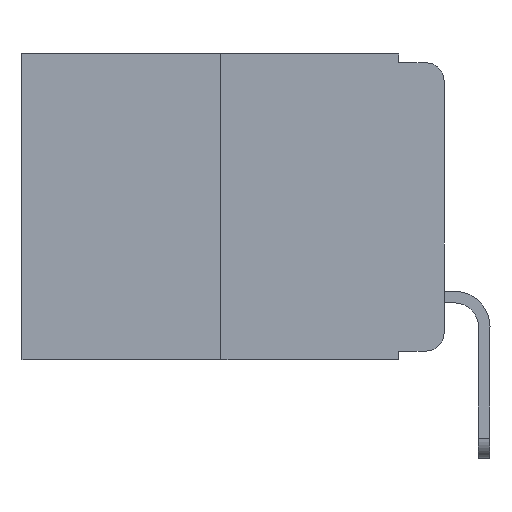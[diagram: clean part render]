
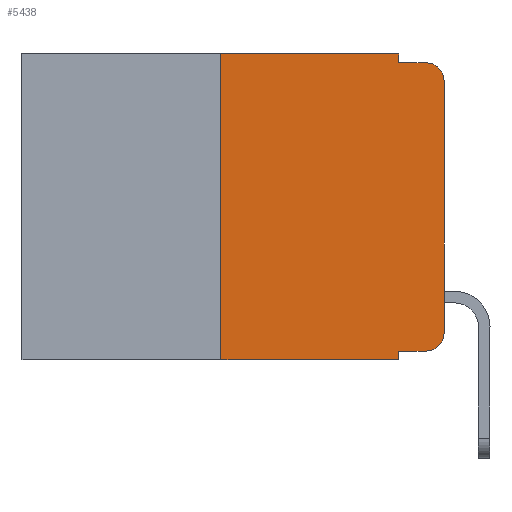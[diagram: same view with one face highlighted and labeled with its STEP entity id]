
A CAD part, left-side view. The second image highlights one B-rep face of the part: STEP entity #5438.
In plain terms, the highlighted planar face has unit normal (-1, 0, 0).
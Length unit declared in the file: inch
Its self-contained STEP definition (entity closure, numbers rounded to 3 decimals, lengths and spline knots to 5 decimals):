
#16 = DIRECTION ( 'NONE',  ( 0., 0., -1. ) ) ;
#187 = CARTESIAN_POINT ( 'NONE',  ( 0., 0., -0.313 ) ) ;
#477 = ORIENTED_EDGE ( 'NONE', *, *, #481, .T. ) ;
#481 = EDGE_CURVE ( 'NONE', #2038, #12820, #4282, .T. ) ;
#696 = EDGE_CURVE ( 'NONE', #2451, #9400, #4997, .T. ) ;
#844 = VERTEX_POINT ( 'NONE', #4598 ) ;
#1097 = CARTESIAN_POINT ( 'NONE',  ( 0., 0.473, -0.343 ) ) ;
#1273 = ORIENTED_EDGE ( 'NONE', *, *, #2085, .T. ) ;
#1280 = VECTOR ( 'NONE', #8300, 39.37008 ) ;
#1400 = LINE ( 'NONE', #3022, #12144 ) ;
#1419 = CARTESIAN_POINT ( 'NONE',  ( 0., 0.473, 0. ) ) ;
#1587 = CARTESIAN_POINT ( 'NONE',  ( 0., 0.25, -0.343 ) ) ;
#1633 = VECTOR ( 'NONE', #10096, 39.37008 ) ;
#1708 = CARTESIAN_POINT ( 'NONE',  ( 0., 0.051, 0. ) ) ;
#1951 = ORIENTED_EDGE ( 'NONE', *, *, #5269, .F. ) ;
#2038 = VERTEX_POINT ( 'NONE', #187 ) ;
#2085 = EDGE_CURVE ( 'NONE', #12820, #3923, #8723, .T. ) ;
#2230 = VERTEX_POINT ( 'NONE', #1587 ) ;
#2451 = VERTEX_POINT ( 'NONE', #7808 ) ;
#2529 = LINE ( 'NONE', #4290, #1633 ) ;
#2653 = VECTOR ( 'NONE', #7726, 39.37008 ) ;
#3007 = FACE_OUTER_BOUND ( 'NONE', #12797, .T. ) ;
#3022 = CARTESIAN_POINT ( 'NONE',  ( 0., 0.051, -0.333 ) ) ;
#3183 = AXIS2_PLACEMENT_3D ( 'NONE', #14115, #6069, #3643 ) ;
#3369 = LINE ( 'NONE', #1419, #11816 ) ;
#3457 = ORIENTED_EDGE ( 'NONE', *, *, #11152, .T. ) ;
#3540 = CARTESIAN_POINT ( 'NONE',  ( 0., 0.02, -0.313 ) ) ;
#3643 = DIRECTION ( 'NONE',  ( 0., 0., -1. ) ) ;
#3923 = VERTEX_POINT ( 'NONE', #4450 ) ;
#4162 = ORIENTED_EDGE ( 'NONE', *, *, #10431, .F. ) ;
#4205 = ORIENTED_EDGE ( 'NONE', *, *, #12530, .F. ) ;
#4282 = LINE ( 'NONE', #14617, #2653 ) ;
#4290 = CARTESIAN_POINT ( 'NONE',  ( 0., 0.051, -0.01 ) ) ;
#4398 = EDGE_CURVE ( 'NONE', #7217, #3923, #2529, .T. ) ;
#4450 = CARTESIAN_POINT ( 'NONE',  ( 0., 0.02, -0.01 ) ) ;
#4598 = CARTESIAN_POINT ( 'NONE',  ( 0., 0.02, -0.333 ) ) ;
#4603 = PLANE ( 'NONE',  #7050 ) ;
#4630 = CIRCLE ( 'NONE', #14713, 0.02 ) ;
#4679 = CARTESIAN_POINT ( 'NONE',  ( 0., 0.25, 0. ) ) ;
#4997 = LINE ( 'NONE', #1708, #12148 ) ;
#5269 = EDGE_CURVE ( 'NONE', #13619, #13014, #3369, .T. ) ;
#5276 = CARTESIAN_POINT ( 'NONE',  ( 0., 0.25, 0. ) ) ;
#5438 = ADVANCED_FACE ( 'NONE', ( #3007 ), #4603, .F. ) ;
#5814 = EDGE_CURVE ( 'NONE', #844, #2038, #4630, .T. ) ;
#6069 = DIRECTION ( 'NONE',  ( -1., 0., 0. ) ) ;
#6144 = LINE ( 'NONE', #4679, #1280 ) ;
#6895 = DIRECTION ( 'NONE',  ( 1., 0., 0. ) ) ;
#7050 = AXIS2_PLACEMENT_3D ( 'NONE', #8214, #6895, #16 ) ;
#7104 = DIRECTION ( 'NONE',  ( -1., 0., 0. ) ) ;
#7217 = VERTEX_POINT ( 'NONE', #9173 ) ;
#7726 = DIRECTION ( 'NONE',  ( 0., 0., 1. ) ) ;
#7808 = CARTESIAN_POINT ( 'NONE',  ( 0., 0.051, -0.333 ) ) ;
#8214 = CARTESIAN_POINT ( 'NONE',  ( 0., 0.473, 0. ) ) ;
#8300 = DIRECTION ( 'NONE',  ( 0., 0., 1. ) ) ;
#8420 = CARTESIAN_POINT ( 'NONE',  ( 0., 0.051, 0. ) ) ;
#8710 = LINE ( 'NONE', #1097, #14581 ) ;
#8723 = CIRCLE ( 'NONE', #3183, 0.02 ) ;
#8981 = LINE ( 'NONE', #8420, #13079 ) ;
#9173 = CARTESIAN_POINT ( 'NONE',  ( 0., 0.051, -0.01 ) ) ;
#9244 = DIRECTION ( 'NONE',  ( 0., -1., 0. ) ) ;
#9356 = ORIENTED_EDGE ( 'NONE', *, *, #696, .F. ) ;
#9400 = VERTEX_POINT ( 'NONE', #9936 ) ;
#9554 = DIRECTION ( 'NONE',  ( 0., 0., -1. ) ) ;
#9936 = CARTESIAN_POINT ( 'NONE',  ( 0., 0.051, -0.343 ) ) ;
#10096 = DIRECTION ( 'NONE',  ( 0., -1., 0. ) ) ;
#10431 = EDGE_CURVE ( 'NONE', #13014, #7217, #8981, .T. ) ;
#10558 = ORIENTED_EDGE ( 'NONE', *, *, #5814, .T. ) ;
#10721 = ORIENTED_EDGE ( 'NONE', *, *, #14336, .T. ) ;
#10815 = DIRECTION ( 'NONE',  ( 0., 0., -1. ) ) ;
#11152 = EDGE_CURVE ( 'NONE', #2230, #9400, #8710, .T. ) ;
#11316 = DIRECTION ( 'NONE',  ( 0., -1., 0. ) ) ;
#11662 = DIRECTION ( 'NONE',  ( 0., 0., -1. ) ) ;
#11816 = VECTOR ( 'NONE', #9244, 39.37008 ) ;
#12144 = VECTOR ( 'NONE', #13391, 39.37008 ) ;
#12148 = VECTOR ( 'NONE', #10815, 39.37008 ) ;
#12530 = EDGE_CURVE ( 'NONE', #2230, #13619, #6144, .T. ) ;
#12797 = EDGE_LOOP ( 'NONE', ( #477, #1273, #13149, #4162, #1951, #4205, #3457, #9356, #10721, #10558 ) ) ;
#12820 = VERTEX_POINT ( 'NONE', #13323 ) ;
#13014 = VERTEX_POINT ( 'NONE', #13378 ) ;
#13079 = VECTOR ( 'NONE', #9554, 39.37008 ) ;
#13149 = ORIENTED_EDGE ( 'NONE', *, *, #4398, .F. ) ;
#13323 = CARTESIAN_POINT ( 'NONE',  ( 0., 0., -0.03 ) ) ;
#13378 = CARTESIAN_POINT ( 'NONE',  ( 0., 0.051, 0. ) ) ;
#13391 = DIRECTION ( 'NONE',  ( 0., -1., 0. ) ) ;
#13619 = VERTEX_POINT ( 'NONE', #5276 ) ;
#14115 = CARTESIAN_POINT ( 'NONE',  ( 0., 0.02, -0.03 ) ) ;
#14336 = EDGE_CURVE ( 'NONE', #2451, #844, #1400, .T. ) ;
#14581 = VECTOR ( 'NONE', #11316, 39.37008 ) ;
#14617 = CARTESIAN_POINT ( 'NONE',  ( 0., 0., 0. ) ) ;
#14713 = AXIS2_PLACEMENT_3D ( 'NONE', #3540, #7104, #11662 ) ;
